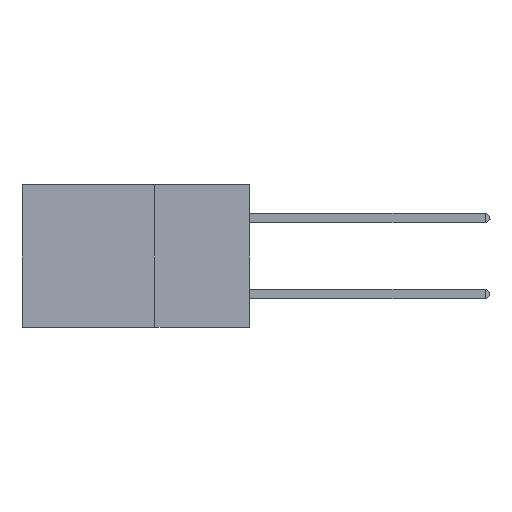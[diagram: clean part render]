
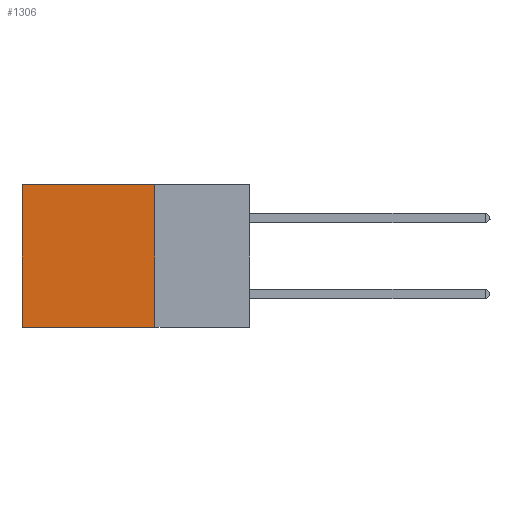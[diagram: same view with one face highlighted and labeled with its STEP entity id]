
A CAD part, left-side view. The second image highlights one B-rep face of the part: STEP entity #1306.
In plain terms, the highlighted planar face has unit normal (-1, 0, 0).
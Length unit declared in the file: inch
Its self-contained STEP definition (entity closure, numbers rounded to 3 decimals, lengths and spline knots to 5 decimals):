
#1208 = CARTESIAN_POINT ( 'NONE',  ( 0.2875, 0.25, -0.375 ) ) ;
#1216 = VECTOR ( 'NONE', #1469, 39.37008 ) ;
#1306 = ADVANCED_FACE ( 'NONE', ( #11540 ), #2344, .F. ) ;
#1337 = EDGE_CURVE ( 'NONE', #6741, #4262, #5959, .T. ) ;
#1469 = DIRECTION ( 'NONE',  ( 0., 0., -1. ) ) ;
#1959 = AXIS2_PLACEMENT_3D ( 'NONE', #1208, #5815, #4752 ) ;
#2344 = PLANE ( 'NONE',  #1959 ) ;
#2441 = ORIENTED_EDGE ( 'NONE', *, *, #11174, .F. ) ;
#2507 = LINE ( 'NONE', #12980, #9456 ) ;
#2988 = LINE ( 'NONE', #12414, #8481 ) ;
#3571 = CARTESIAN_POINT ( 'NONE',  ( 0.2875, 0.6, -0.375 ) ) ;
#4262 = VERTEX_POINT ( 'NONE', #14490 ) ;
#4681 = CARTESIAN_POINT ( 'NONE',  ( 0.2875, 0.25, 0. ) ) ;
#4752 = DIRECTION ( 'NONE',  ( 0., 0., -1. ) ) ;
#5321 = EDGE_CURVE ( 'NONE', #4262, #14119, #8391, .T. ) ;
#5815 = DIRECTION ( 'NONE',  ( 1., 0., 0. ) ) ;
#5959 = LINE ( 'NONE', #4681, #13727 ) ;
#6741 = VERTEX_POINT ( 'NONE', #8343 ) ;
#7109 = DIRECTION ( 'NONE',  ( 0., 1., 0. ) ) ;
#7145 = CARTESIAN_POINT ( 'NONE',  ( 0.2875, 0.6, -0.375 ) ) ;
#7726 = DIRECTION ( 'NONE',  ( 0., 0., -1. ) ) ;
#7889 = CARTESIAN_POINT ( 'NONE',  ( 0.2875, 0.25, -0.375 ) ) ;
#8343 = CARTESIAN_POINT ( 'NONE',  ( 0.2875, 0.25, 0. ) ) ;
#8391 = LINE ( 'NONE', #3571, #1216 ) ;
#8457 = ORIENTED_EDGE ( 'NONE', *, *, #5321, .T. ) ;
#8481 = VECTOR ( 'NONE', #7726, 39.37008 ) ;
#9456 = VECTOR ( 'NONE', #7109, 39.37008 ) ;
#9966 = ORIENTED_EDGE ( 'NONE', *, *, #13287, .F. ) ;
#10945 = ORIENTED_EDGE ( 'NONE', *, *, #1337, .T. ) ;
#11174 = EDGE_CURVE ( 'NONE', #6741, #14507, #2988, .T. ) ;
#11540 = FACE_OUTER_BOUND ( 'NONE', #13404, .T. ) ;
#12414 = CARTESIAN_POINT ( 'NONE',  ( 0.2875, 0.25, -0.375 ) ) ;
#12980 = CARTESIAN_POINT ( 'NONE',  ( 0.2875, 0.25, -0.375 ) ) ;
#13287 = EDGE_CURVE ( 'NONE', #14507, #14119, #2507, .T. ) ;
#13404 = EDGE_LOOP ( 'NONE', ( #8457, #9966, #2441, #10945 ) ) ;
#13725 = DIRECTION ( 'NONE',  ( 0., 1., 0. ) ) ;
#13727 = VECTOR ( 'NONE', #13725, 39.37008 ) ;
#14119 = VERTEX_POINT ( 'NONE', #7145 ) ;
#14490 = CARTESIAN_POINT ( 'NONE',  ( 0.2875, 0.6, 0. ) ) ;
#14507 = VERTEX_POINT ( 'NONE', #7889 ) ;
